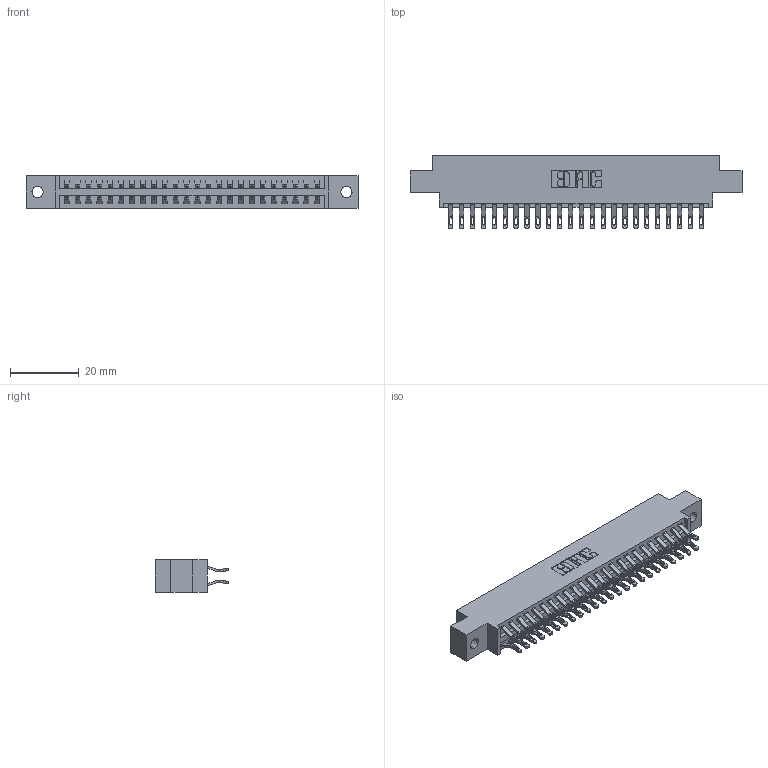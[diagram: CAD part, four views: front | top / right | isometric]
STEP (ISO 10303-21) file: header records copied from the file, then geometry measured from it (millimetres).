
FILE_DESCRIPTION (( 'STEP AP203' ), '1' );
FILE_NAME ('396-048-555-802.STEP', '2018-09-08T00:38:47', ( '' ), ( '' ), 'SwSTEP 2.0', 'SolidWorks 2016', '' );
FILE_SCHEMA (( 'CONFIG_CONTROL_DESIGN' ));
Length unit declared in the file: inch
Products named in the file (3): 346 Part_0.170 Offset - 0.128 Dia; 345-292-001_555 Tail; 396-048-555-802
Assembly tree (49 placements, depth 2):
  396-048-555-802
    346 Part_0.170 Offset - 0.128 Dia
    345-292-001_555 Tail  x48
Bounding box: 96.77 x 21.46 x 9.4 mm (x, y, z)
Volume: 9244.8 mm3; surface area: 12831.3 mm2
Topology: 49 solids, 49 shells, 2910 faces, 9125 edges, 6082 vertices
Faces by surface type: plane 1664, cylinder 1246
Entity records: 18547 total; most frequent: CARTESIAN_POINT 3118, ORIENTED_EDGE 3022, DIRECTION 2767, EDGE_CURVE 1511, VECTOR 1263, LINE 1263, VERTEX_POINT 1006, AXIS2_PLACEMENT_3D 752
